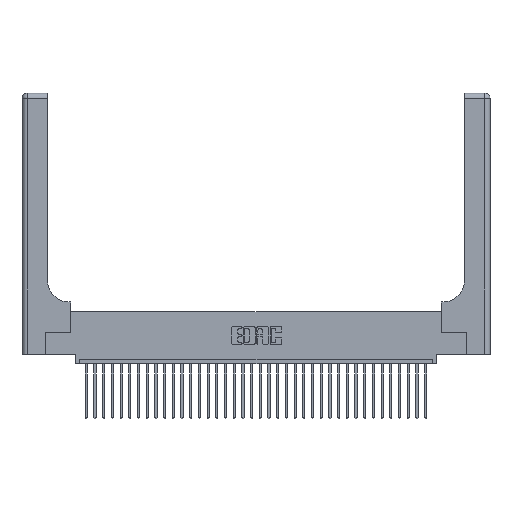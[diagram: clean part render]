
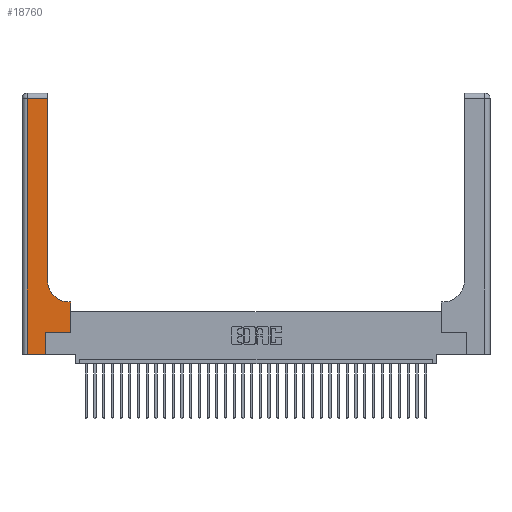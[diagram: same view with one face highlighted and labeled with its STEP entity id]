
A CAD part, top view. The second image highlights one B-rep face of the part: STEP entity #18760.
In plain terms, the highlighted planar face has unit normal (0, 0, 1).
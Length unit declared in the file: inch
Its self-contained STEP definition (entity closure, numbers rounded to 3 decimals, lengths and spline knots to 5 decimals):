
#54 = ORIENTED_EDGE ( 'NONE', *, *, #21978, .T. ) ;
#166 = CARTESIAN_POINT ( 'NONE',  ( 0.2915, 3., 0.37 ) ) ;
#225 = DIRECTION ( 'NONE',  ( 0., 0., -1. ) ) ;
#273 = DIRECTION ( 'NONE',  ( 0., 0., -1. ) ) ;
#375 = VECTOR ( 'NONE', #29111, 39.37008 ) ;
#1034 = ORIENTED_EDGE ( 'NONE', *, *, #5621, .T. ) ;
#1835 = VERTEX_POINT ( 'NONE', #26501 ) ;
#2447 = CARTESIAN_POINT ( 'NONE',  ( 0.06, 0., 0.37 ) ) ;
#2726 = VECTOR ( 'NONE', #21877, 39.37008 ) ;
#2871 = VERTEX_POINT ( 'NONE', #6407 ) ;
#3172 = VECTOR ( 'NONE', #28133, 39.37008 ) ;
#4747 = FACE_OUTER_BOUND ( 'NONE', #20987, .T. ) ;
#4885 = VERTEX_POINT ( 'NONE', #22890 ) ;
#5350 = VECTOR ( 'NONE', #20134, 39.37008 ) ;
#5419 = DIRECTION ( 'NONE',  ( 0., 1., 0. ) ) ;
#5621 = EDGE_CURVE ( 'NONE', #28412, #4885, #25172, .T. ) ;
#5636 = CARTESIAN_POINT ( 'NONE',  ( 0.5585, 0.25, 0.37 ) ) ;
#5887 = CIRCLE ( 'NONE', #14088, 0.25 ) ;
#6407 = CARTESIAN_POINT ( 'NONE',  ( 0.269, 0.25, 0.37 ) ) ;
#6800 = ORIENTED_EDGE ( 'NONE', *, *, #33606, .T. ) ;
#7365 = LINE ( 'NONE', #35007, #375 ) ;
#7881 = ORIENTED_EDGE ( 'NONE', *, *, #20653, .T. ) ;
#8177 = PLANE ( 'NONE',  #27300 ) ;
#8562 = CARTESIAN_POINT ( 'NONE',  ( 0.5415, 0.85, 0.37 ) ) ;
#9696 = LINE ( 'NONE', #11928, #5350 ) ;
#9857 = CARTESIAN_POINT ( 'NONE',  ( 0.2915, 2.94, 0.37 ) ) ;
#10154 = VERTEX_POINT ( 'NONE', #28143 ) ;
#10267 = VERTEX_POINT ( 'NONE', #9857 ) ;
#10697 = CARTESIAN_POINT ( 'NONE',  ( 0.2915, 0.6, 0.37 ) ) ;
#11240 = DIRECTION ( 'NONE',  ( -1., 0., 0. ) ) ;
#11672 = CARTESIAN_POINT ( 'NONE',  ( 0.5585, 0.25, 0.37 ) ) ;
#11928 = CARTESIAN_POINT ( 'NONE',  ( 0.269, 0., 0.37 ) ) ;
#11961 = ORIENTED_EDGE ( 'NONE', *, *, #31258, .T. ) ;
#14088 = AXIS2_PLACEMENT_3D ( 'NONE', #8562, #225, #22739 ) ;
#14212 = VECTOR ( 'NONE', #30446, 39.37008 ) ;
#16201 = ORIENTED_EDGE ( 'NONE', *, *, #23058, .T. ) ;
#16557 = CARTESIAN_POINT ( 'NONE',  ( 0., 3., 0.37 ) ) ;
#17800 = EDGE_CURVE ( 'NONE', #21032, #10154, #17930, .T. ) ;
#17838 = VECTOR ( 'NONE', #11240, 39.37008 ) ;
#17930 = LINE ( 'NONE', #10697, #3172 ) ;
#18093 = VERTEX_POINT ( 'NONE', #30577 ) ;
#18217 = CARTESIAN_POINT ( 'NONE',  ( 0.269, 0.25, 0.37 ) ) ;
#18760 = ADVANCED_FACE ( 'NONE', ( #4747 ), #8177, .F. ) ;
#19063 = ORIENTED_EDGE ( 'NONE', *, *, #33001, .T. ) ;
#20019 = ORIENTED_EDGE ( 'NONE', *, *, #17800, .T. ) ;
#20134 = DIRECTION ( 'NONE',  ( 0., 1., 0. ) ) ;
#20625 = ORIENTED_EDGE ( 'NONE', *, *, #35630, .T. ) ;
#20653 = EDGE_CURVE ( 'NONE', #2871, #22125, #23638, .T. ) ;
#20987 = EDGE_LOOP ( 'NONE', ( #20625, #16201, #11961, #1034, #54, #7881, #6800, #20019, #19063 ) ) ;
#21032 = VERTEX_POINT ( 'NONE', #22545 ) ;
#21501 = VECTOR ( 'NONE', #5419, 39.37008 ) ;
#21877 = DIRECTION ( 'NONE',  ( 1., 0., 0. ) ) ;
#21978 = EDGE_CURVE ( 'NONE', #4885, #2871, #9696, .T. ) ;
#22125 = VERTEX_POINT ( 'NONE', #11672 ) ;
#22545 = CARTESIAN_POINT ( 'NONE',  ( 0.5585, 0.6, 0.37 ) ) ;
#22739 = DIRECTION ( 'NONE',  ( 1., 0., 0. ) ) ;
#22890 = CARTESIAN_POINT ( 'NONE',  ( 0.269, 0., 0.37 ) ) ;
#23058 = EDGE_CURVE ( 'NONE', #10267, #18093, #27327, .T. ) ;
#23638 = LINE ( 'NONE', #18217, #35667 ) ;
#24522 = CARTESIAN_POINT ( 'NONE',  ( 0., 0., 0.37 ) ) ;
#25036 = DIRECTION ( 'NONE',  ( 1., 0., 0. ) ) ;
#25172 = LINE ( 'NONE', #24522, #2726 ) ;
#26501 = CARTESIAN_POINT ( 'NONE',  ( 0.2915, 0.85, 0.37 ) ) ;
#27142 = LINE ( 'NONE', #166, #14212 ) ;
#27300 = AXIS2_PLACEMENT_3D ( 'NONE', #16557, #273, #33225 ) ;
#27327 = LINE ( 'NONE', #27771, #17838 ) ;
#27771 = CARTESIAN_POINT ( 'NONE',  ( 0., 2.94, 0.37 ) ) ;
#28133 = DIRECTION ( 'NONE',  ( -1., 0., 0. ) ) ;
#28143 = CARTESIAN_POINT ( 'NONE',  ( 0.5415, 0.6, 0.37 ) ) ;
#28412 = VERTEX_POINT ( 'NONE', #2447 ) ;
#28790 = LINE ( 'NONE', #5636, #21501 ) ;
#29111 = DIRECTION ( 'NONE',  ( 0., -1., 0. ) ) ;
#30446 = DIRECTION ( 'NONE',  ( 0., 1., 0. ) ) ;
#30577 = CARTESIAN_POINT ( 'NONE',  ( 0.06, 2.94, 0.37 ) ) ;
#31258 = EDGE_CURVE ( 'NONE', #18093, #28412, #7365, .T. ) ;
#33001 = EDGE_CURVE ( 'NONE', #10154, #1835, #5887, .T. ) ;
#33225 = DIRECTION ( 'NONE',  ( -1., 0., 0. ) ) ;
#33606 = EDGE_CURVE ( 'NONE', #22125, #21032, #28790, .T. ) ;
#35007 = CARTESIAN_POINT ( 'NONE',  ( 0.06, 3., 0.37 ) ) ;
#35630 = EDGE_CURVE ( 'NONE', #1835, #10267, #27142, .T. ) ;
#35667 = VECTOR ( 'NONE', #25036, 39.37008 ) ;
